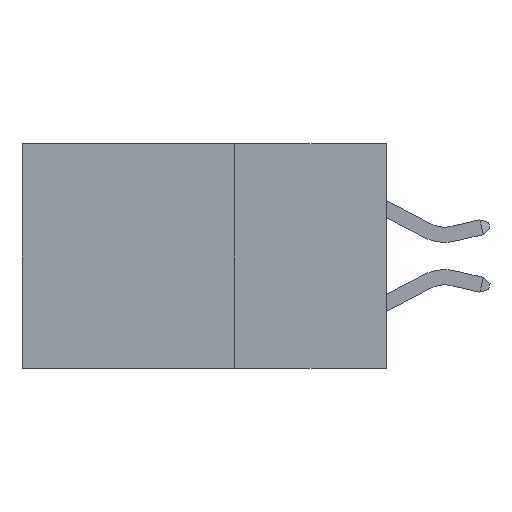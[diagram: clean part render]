
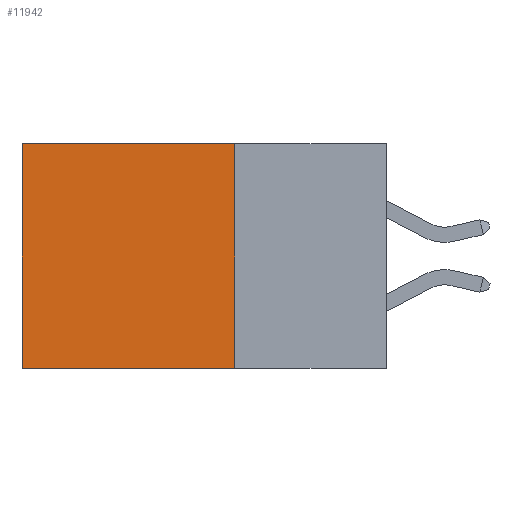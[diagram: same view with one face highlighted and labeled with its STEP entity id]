
A CAD part, left-side view. The second image highlights one B-rep face of the part: STEP entity #11942.
In plain terms, the highlighted planar face has unit normal (-1, 0, 0).
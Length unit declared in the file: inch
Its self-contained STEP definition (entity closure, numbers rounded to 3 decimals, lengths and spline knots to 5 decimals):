
#562 = CARTESIAN_POINT ( 'NONE',  ( 0.2615, 0.6, 0. ) ) ;
#1247 = CARTESIAN_POINT ( 'NONE',  ( 0.2615, 0.6, -0.37 ) ) ;
#1373 = EDGE_CURVE ( 'NONE', #10011, #6562, #8415, .T. ) ;
#4060 = EDGE_CURVE ( 'NONE', #6562, #5458, #11381, .T. ) ;
#4408 = CARTESIAN_POINT ( 'NONE',  ( 0.2615, 0.25, 0. ) ) ;
#5458 = VERTEX_POINT ( 'NONE', #13618 ) ;
#6562 = VERTEX_POINT ( 'NONE', #11324 ) ;
#6791 = AXIS2_PLACEMENT_3D ( 'NONE', #14138, #14087, #14060 ) ;
#7540 = ORIENTED_EDGE ( 'NONE', *, *, #10843, .T. ) ;
#7899 = ORIENTED_EDGE ( 'NONE', *, *, #8857, .T. ) ;
#8415 = LINE ( 'NONE', #12120, #13953 ) ;
#8857 = EDGE_CURVE ( 'NONE', #10011, #11728, #14368, .T. ) ;
#9560 = FACE_OUTER_BOUND ( 'NONE', #13278, .T. ) ;
#10011 = VERTEX_POINT ( 'NONE', #4408 ) ;
#10124 = VECTOR ( 'NONE', #14822, 39.37008 ) ;
#10597 = ORIENTED_EDGE ( 'NONE', *, *, #4060, .F. ) ;
#10843 = EDGE_CURVE ( 'NONE', #11728, #5458, #13091, .T. ) ;
#10993 = CARTESIAN_POINT ( 'NONE',  ( 0.2615, 0.25, -0.37 ) ) ;
#11013 = VECTOR ( 'NONE', #11062, 39.37008 ) ;
#11062 = DIRECTION ( 'NONE',  ( 0., 1., 0. ) ) ;
#11324 = CARTESIAN_POINT ( 'NONE',  ( 0.2615, 0.25, -0.37 ) ) ;
#11381 = LINE ( 'NONE', #10993, #11013 ) ;
#11646 = DIRECTION ( 'NONE',  ( 0., 1., 0. ) ) ;
#11671 = CARTESIAN_POINT ( 'NONE',  ( 0.2615, 0.25, 0. ) ) ;
#11728 = VERTEX_POINT ( 'NONE', #562 ) ;
#11942 = ADVANCED_FACE ( 'NONE', ( #9560 ), #14121, .F. ) ;
#11966 = VECTOR ( 'NONE', #11646, 39.37008 ) ;
#11978 = DIRECTION ( 'NONE',  ( 0., 0., -1. ) ) ;
#12120 = CARTESIAN_POINT ( 'NONE',  ( 0.2615, 0.25, -0.37 ) ) ;
#13091 = LINE ( 'NONE', #1247, #10124 ) ;
#13278 = EDGE_LOOP ( 'NONE', ( #7540, #10597, #13494, #7899 ) ) ;
#13494 = ORIENTED_EDGE ( 'NONE', *, *, #1373, .F. ) ;
#13618 = CARTESIAN_POINT ( 'NONE',  ( 0.2615, 0.6, -0.37 ) ) ;
#13953 = VECTOR ( 'NONE', #11978, 39.37008 ) ;
#14060 = DIRECTION ( 'NONE',  ( 0., 0., -1. ) ) ;
#14087 = DIRECTION ( 'NONE',  ( 1., 0., 0. ) ) ;
#14121 = PLANE ( 'NONE',  #6791 ) ;
#14138 = CARTESIAN_POINT ( 'NONE',  ( 0.2615, 0.25, -0.37 ) ) ;
#14368 = LINE ( 'NONE', #11671, #11966 ) ;
#14822 = DIRECTION ( 'NONE',  ( 0., 0., -1. ) ) ;
